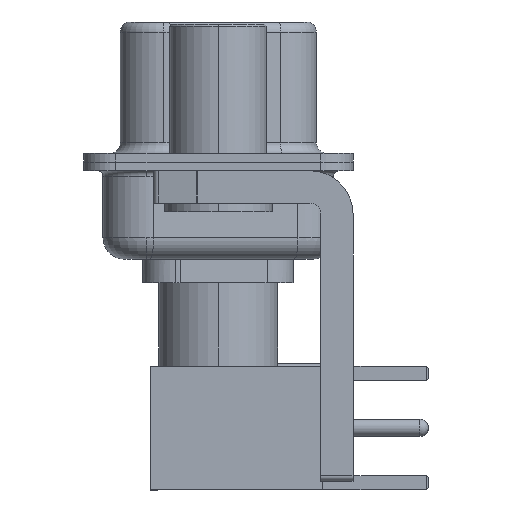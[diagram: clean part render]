
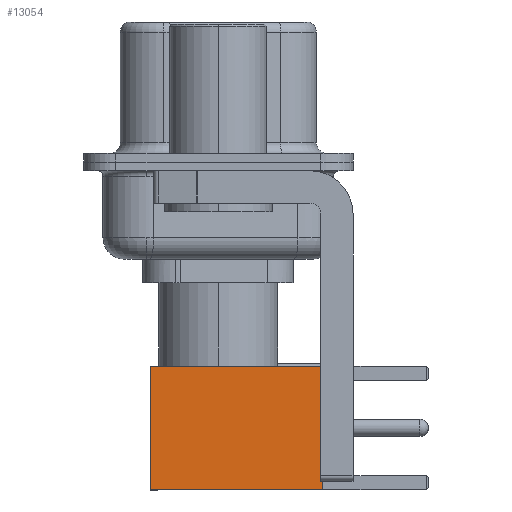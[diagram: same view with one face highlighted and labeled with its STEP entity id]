
A CAD part, left-side view. The second image highlights one B-rep face of the part: STEP entity #13054.
In plain terms, the highlighted face is planar.
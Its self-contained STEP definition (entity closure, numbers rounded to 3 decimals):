
#628 = LINE ( 'NONE', #11017, #24579 ) ;
#921 = AXIS2_PLACEMENT_3D ( 'NONE', #17354, #25900, #15097 ) ;
#1253 = ORIENTED_EDGE ( 'NONE', *, *, #13414, .F. ) ;
#2021 = CARTESIAN_POINT ( 'NONE',  ( 2.875, 2.875, 0. ) ) ;
#3455 = CARTESIAN_POINT ( 'NONE',  ( -2.875, 2.875, 0. ) ) ;
#5661 = VERTEX_POINT ( 'NONE', #11724 ) ;
#7402 = EDGE_LOOP ( 'NONE', ( #15944, #24547, #14698, #1253 ) ) ;
#8357 = CARTESIAN_POINT ( 'NONE',  ( -2.875, 2.875, 0. ) ) ;
#8911 = EDGE_CURVE ( 'NONE', #18529, #26294, #628, .T. ) ;
#10769 = VECTOR ( 'NONE', #27434, 1000. ) ;
#11017 = CARTESIAN_POINT ( 'NONE',  ( 0., 2.875, 0. ) ) ;
#11724 = CARTESIAN_POINT ( 'NONE',  ( -2.875, 2.875, 8. ) ) ;
#12898 = EDGE_CURVE ( 'NONE', #5661, #26294, #16638, .T. ) ;
#13054 = ADVANCED_FACE ( 'NONE', ( #21836 ), #17486, .T. ) ;
#13414 = EDGE_CURVE ( 'NONE', #21924, #5661, #25466, .T. ) ;
#14698 = ORIENTED_EDGE ( 'NONE', *, *, #12898, .F. ) ;
#15097 = DIRECTION ( 'NONE',  ( 0., 0., 1. ) ) ;
#15183 = CARTESIAN_POINT ( 'NONE',  ( 2.875, 2.875, 0. ) ) ;
#15944 = ORIENTED_EDGE ( 'NONE', *, *, #24589, .T. ) ;
#16638 = LINE ( 'NONE', #8357, #10769 ) ;
#17354 = CARTESIAN_POINT ( 'NONE',  ( 2.875, 2.875, 0. ) ) ;
#17486 = PLANE ( 'NONE',  #921 ) ;
#18529 = VERTEX_POINT ( 'NONE', #2021 ) ;
#19179 = DIRECTION ( 'NONE',  ( -1., 0., 0. ) ) ;
#19773 = VECTOR ( 'NONE', #19179, 1000. ) ;
#19850 = DIRECTION ( 'NONE',  ( -1., 0., 0. ) ) ;
#21836 = FACE_OUTER_BOUND ( 'NONE', #7402, .T. ) ;
#21924 = VERTEX_POINT ( 'NONE', #26098 ) ;
#23366 = CARTESIAN_POINT ( 'NONE',  ( 0., 2.875, 8. ) ) ;
#23736 = DIRECTION ( 'NONE',  ( 0., 0., -1. ) ) ;
#24547 = ORIENTED_EDGE ( 'NONE', *, *, #8911, .T. ) ;
#24579 = VECTOR ( 'NONE', #19850, 1000. ) ;
#24589 = EDGE_CURVE ( 'NONE', #21924, #18529, #25837, .T. ) ;
#25466 = LINE ( 'NONE', #23366, #19773 ) ;
#25837 = LINE ( 'NONE', #15183, #26874 ) ;
#25900 = DIRECTION ( 'NONE',  ( 0., 1., 0. ) ) ;
#26098 = CARTESIAN_POINT ( 'NONE',  ( 2.875, 2.875, 8. ) ) ;
#26294 = VERTEX_POINT ( 'NONE', #3455 ) ;
#26874 = VECTOR ( 'NONE', #23736, 1000. ) ;
#27434 = DIRECTION ( 'NONE',  ( 0., 0., -1. ) ) ;
